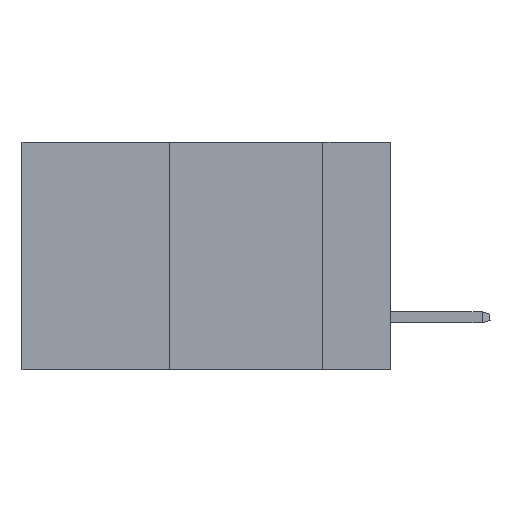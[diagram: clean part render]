
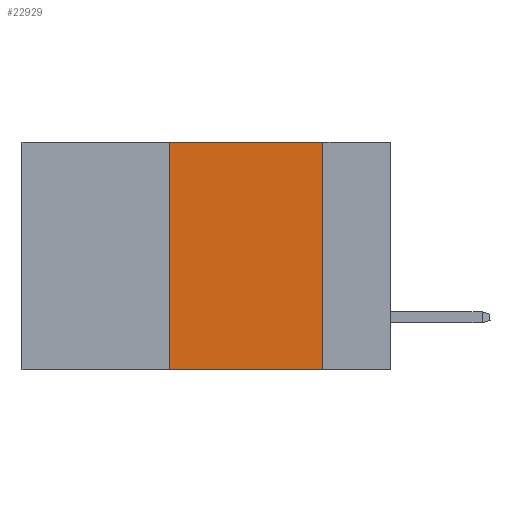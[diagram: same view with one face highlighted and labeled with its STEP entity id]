
A CAD part, left-side view. The second image highlights one B-rep face of the part: STEP entity #22929.
In plain terms, the highlighted planar face has unit normal (-1, 0, 0).
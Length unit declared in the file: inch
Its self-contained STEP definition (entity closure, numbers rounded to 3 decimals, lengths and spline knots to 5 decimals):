
#703 = VECTOR ( 'NONE', #38267, 39.37008 ) ;
#2456 = CARTESIAN_POINT ( 'NONE',  ( 0., 0.6, -0.37 ) ) ;
#5188 = VERTEX_POINT ( 'NONE', #46070 ) ;
#5583 = EDGE_LOOP ( 'NONE', ( #22370, #8792, #7012, #9424 ) ) ;
#6189 = LINE ( 'NONE', #10764, #37710 ) ;
#6956 = VERTEX_POINT ( 'NONE', #41411 ) ;
#7012 = ORIENTED_EDGE ( 'NONE', *, *, #41561, .F. ) ;
#8698 = CARTESIAN_POINT ( 'NONE',  ( 0., 0.6, 0. ) ) ;
#8792 = ORIENTED_EDGE ( 'NONE', *, *, #41545, .F. ) ;
#8930 = VECTOR ( 'NONE', #40773, 39.37008 ) ;
#9235 = CARTESIAN_POINT ( 'NONE',  ( 0., 0.11, 0. ) ) ;
#9424 = ORIENTED_EDGE ( 'NONE', *, *, #14373, .T. ) ;
#9445 = VERTEX_POINT ( 'NONE', #13570 ) ;
#9992 = VECTOR ( 'NONE', #27584, 39.37008 ) ;
#10764 = CARTESIAN_POINT ( 'NONE',  ( 0., 0.6, 0. ) ) ;
#13570 = CARTESIAN_POINT ( 'NONE',  ( 0., 0.36, 0. ) ) ;
#14373 = EDGE_CURVE ( 'NONE', #5188, #15468, #29133, .T. ) ;
#15468 = VERTEX_POINT ( 'NONE', #39956 ) ;
#15830 = FACE_OUTER_BOUND ( 'NONE', #5583, .T. ) ;
#18780 = CARTESIAN_POINT ( 'NONE',  ( 0., 0.36, 0. ) ) ;
#19462 = DIRECTION ( 'NONE',  ( 1., 0., 0. ) ) ;
#22370 = ORIENTED_EDGE ( 'NONE', *, *, #28458, .F. ) ;
#22929 = ADVANCED_FACE ( 'NONE', ( #15830 ), #37873, .F. ) ;
#27584 = DIRECTION ( 'NONE',  ( 0., -1., 0. ) ) ;
#28458 = EDGE_CURVE ( 'NONE', #6956, #15468, #29340, .T. ) ;
#28899 = DIRECTION ( 'NONE',  ( 0., -1., 0. ) ) ;
#29133 = LINE ( 'NONE', #2456, #9992 ) ;
#29340 = LINE ( 'NONE', #9235, #703 ) ;
#30250 = DIRECTION ( 'NONE',  ( 0., 0., -1. ) ) ;
#34747 = AXIS2_PLACEMENT_3D ( 'NONE', #8698, #19462, #30250 ) ;
#37710 = VECTOR ( 'NONE', #28899, 39.37008 ) ;
#37873 = PLANE ( 'NONE',  #34747 ) ;
#38267 = DIRECTION ( 'NONE',  ( 0., 0., -1. ) ) ;
#38875 = LINE ( 'NONE', #18780, #8930 ) ;
#39956 = CARTESIAN_POINT ( 'NONE',  ( 0., 0.11, -0.37 ) ) ;
#40773 = DIRECTION ( 'NONE',  ( 0., 0., 1. ) ) ;
#41411 = CARTESIAN_POINT ( 'NONE',  ( 0., 0.11, 0. ) ) ;
#41545 = EDGE_CURVE ( 'NONE', #9445, #6956, #6189, .T. ) ;
#41561 = EDGE_CURVE ( 'NONE', #5188, #9445, #38875, .T. ) ;
#46070 = CARTESIAN_POINT ( 'NONE',  ( 0., 0.36, -0.37 ) ) ;
